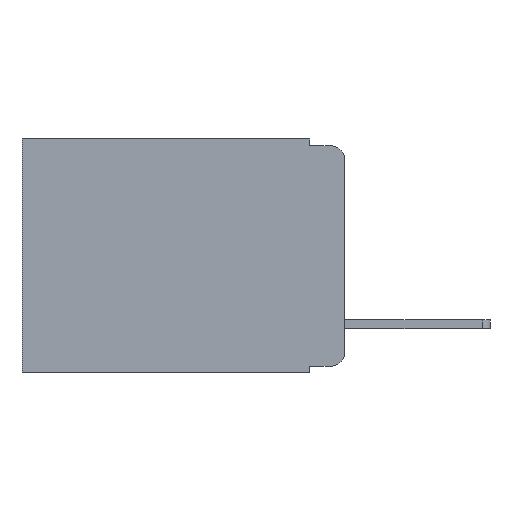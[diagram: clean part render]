
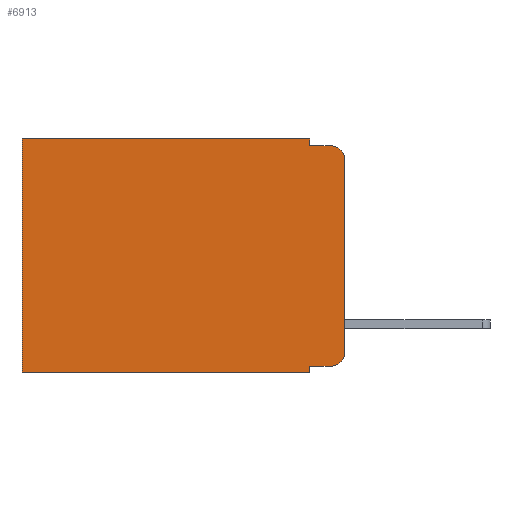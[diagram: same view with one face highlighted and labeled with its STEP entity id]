
A CAD part, left-side view. The second image highlights one B-rep face of the part: STEP entity #6913.
In plain terms, the highlighted planar face has unit normal (-1, 0, 0).
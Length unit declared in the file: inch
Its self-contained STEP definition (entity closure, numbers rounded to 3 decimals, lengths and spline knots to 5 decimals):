
#239 = CARTESIAN_POINT ( 'NONE',  ( 0.298, 0., -0.03 ) ) ;
#267 = VERTEX_POINT ( 'NONE', #1591 ) ;
#398 = CARTESIAN_POINT ( 'NONE',  ( 0.298, 0.473, -0.343 ) ) ;
#424 = DIRECTION ( 'NONE',  ( 0., 1., 0. ) ) ;
#468 = VERTEX_POINT ( 'NONE', #10323 ) ;
#491 = EDGE_CURVE ( 'NONE', #6999, #267, #5347, .T. ) ;
#608 = ORIENTED_EDGE ( 'NONE', *, *, #491, .F. ) ;
#833 = VERTEX_POINT ( 'NONE', #9788 ) ;
#891 = ORIENTED_EDGE ( 'NONE', *, *, #2129, .F. ) ;
#892 = EDGE_CURVE ( 'NONE', #4839, #3375, #2151, .T. ) ;
#1112 = CARTESIAN_POINT ( 'NONE',  ( 0.298, 0., 0. ) ) ;
#1186 = FACE_OUTER_BOUND ( 'NONE', #6972, .T. ) ;
#1490 = ORIENTED_EDGE ( 'NONE', *, *, #1533, .F. ) ;
#1533 = EDGE_CURVE ( 'NONE', #4839, #833, #5191, .T. ) ;
#1591 = CARTESIAN_POINT ( 'NONE',  ( 0.298, 0.051, -0.01 ) ) ;
#1706 = PLANE ( 'NONE',  #8414 ) ;
#1977 = VERTEX_POINT ( 'NONE', #5112 ) ;
#2122 = DIRECTION ( 'NONE',  ( 0., 0., -1. ) ) ;
#2129 = EDGE_CURVE ( 'NONE', #267, #3375, #2554, .T. ) ;
#2151 = CIRCLE ( 'NONE', #7015, 0.02 ) ;
#2209 = CARTESIAN_POINT ( 'NONE',  ( 0.298, 0.051, 0. ) ) ;
#2267 = VECTOR ( 'NONE', #5740, 39.37008 ) ;
#2313 = CARTESIAN_POINT ( 'NONE',  ( 0.298, 0.02, -0.01 ) ) ;
#2428 = EDGE_CURVE ( 'NONE', #1977, #8371, #8918, .T. ) ;
#2472 = AXIS2_PLACEMENT_3D ( 'NONE', #9512, #4552, #10283 ) ;
#2554 = LINE ( 'NONE', #5595, #2267 ) ;
#2742 = CARTESIAN_POINT ( 'NONE',  ( 0.298, 0.051, -0.343 ) ) ;
#2874 = CARTESIAN_POINT ( 'NONE',  ( 0.298, 0., -0.343 ) ) ;
#2921 = LINE ( 'NONE', #2874, #9117 ) ;
#2930 = DIRECTION ( 'NONE',  ( 0., 1., 0. ) ) ;
#3375 = VERTEX_POINT ( 'NONE', #2313 ) ;
#3522 = DIRECTION ( 'NONE',  ( 1., 0., 0. ) ) ;
#3586 = ORIENTED_EDGE ( 'NONE', *, *, #9559, .T. ) ;
#4040 = LINE ( 'NONE', #1112, #6050 ) ;
#4150 = ORIENTED_EDGE ( 'NONE', *, *, #2428, .T. ) ;
#4177 = LINE ( 'NONE', #6265, #5916 ) ;
#4307 = VERTEX_POINT ( 'NONE', #2742 ) ;
#4310 = CARTESIAN_POINT ( 'NONE',  ( 0.298, 0.02, -0.03 ) ) ;
#4516 = DIRECTION ( 'NONE',  ( -1., 0., 0. ) ) ;
#4552 = DIRECTION ( 'NONE',  ( -1., 0., 0. ) ) ;
#4726 = EDGE_CURVE ( 'NONE', #468, #5786, #6727, .T. ) ;
#4756 = VECTOR ( 'NONE', #7923, 39.37008 ) ;
#4793 = EDGE_CURVE ( 'NONE', #468, #4307, #4177, .T. ) ;
#4801 = CIRCLE ( 'NONE', #2472, 0.02 ) ;
#4820 = ORIENTED_EDGE ( 'NONE', *, *, #892, .T. ) ;
#4839 = VERTEX_POINT ( 'NONE', #239 ) ;
#4857 = CARTESIAN_POINT ( 'NONE',  ( 0.298, 0.051, -0.333 ) ) ;
#4916 = VECTOR ( 'NONE', #10443, 39.37008 ) ;
#5079 = VECTOR ( 'NONE', #2122, 39.37008 ) ;
#5112 = CARTESIAN_POINT ( 'NONE',  ( 0.298, 0.473, 0. ) ) ;
#5191 = LINE ( 'NONE', #10582, #4916 ) ;
#5245 = ORIENTED_EDGE ( 'NONE', *, *, #5598, .F. ) ;
#5347 = LINE ( 'NONE', #2209, #5079 ) ;
#5356 = CARTESIAN_POINT ( 'NONE',  ( 0.298, 0.051, 0. ) ) ;
#5595 = CARTESIAN_POINT ( 'NONE',  ( 0.298, 0.051, -0.01 ) ) ;
#5598 = EDGE_CURVE ( 'NONE', #4307, #8371, #2921, .T. ) ;
#5740 = DIRECTION ( 'NONE',  ( 0., -1., 0. ) ) ;
#5786 = VERTEX_POINT ( 'NONE', #8382 ) ;
#5916 = VECTOR ( 'NONE', #6280, 39.37008 ) ;
#6046 = CARTESIAN_POINT ( 'NONE',  ( 0.298, 0., 0. ) ) ;
#6050 = VECTOR ( 'NONE', #2930, 39.37008 ) ;
#6265 = CARTESIAN_POINT ( 'NONE',  ( 0.298, 0.051, 0. ) ) ;
#6280 = DIRECTION ( 'NONE',  ( 0., 0., -1. ) ) ;
#6727 = LINE ( 'NONE', #4857, #8616 ) ;
#6784 = CARTESIAN_POINT ( 'NONE',  ( 0.298, 0.473, 0. ) ) ;
#6913 = ADVANCED_FACE ( 'NONE', ( #1186 ), #1706, .F. ) ;
#6972 = EDGE_LOOP ( 'NONE', ( #1490, #4820, #891, #608, #3586, #4150, #5245, #9341, #9851, #8982 ) ) ;
#6999 = VERTEX_POINT ( 'NONE', #5356 ) ;
#7013 = EDGE_CURVE ( 'NONE', #5786, #833, #4801, .T. ) ;
#7015 = AXIS2_PLACEMENT_3D ( 'NONE', #4310, #4516, #10715 ) ;
#7923 = DIRECTION ( 'NONE',  ( 0., 0., -1. ) ) ;
#8371 = VERTEX_POINT ( 'NONE', #398 ) ;
#8382 = CARTESIAN_POINT ( 'NONE',  ( 0.298, 0.02, -0.333 ) ) ;
#8414 = AXIS2_PLACEMENT_3D ( 'NONE', #6046, #3522, #9370 ) ;
#8616 = VECTOR ( 'NONE', #10179, 39.37008 ) ;
#8918 = LINE ( 'NONE', #6784, #4756 ) ;
#8982 = ORIENTED_EDGE ( 'NONE', *, *, #7013, .T. ) ;
#9117 = VECTOR ( 'NONE', #424, 39.37008 ) ;
#9341 = ORIENTED_EDGE ( 'NONE', *, *, #4793, .F. ) ;
#9370 = DIRECTION ( 'NONE',  ( 0., 0., -1. ) ) ;
#9512 = CARTESIAN_POINT ( 'NONE',  ( 0.298, 0.02, -0.313 ) ) ;
#9559 = EDGE_CURVE ( 'NONE', #6999, #1977, #4040, .T. ) ;
#9788 = CARTESIAN_POINT ( 'NONE',  ( 0.298, 0., -0.313 ) ) ;
#9851 = ORIENTED_EDGE ( 'NONE', *, *, #4726, .T. ) ;
#10179 = DIRECTION ( 'NONE',  ( 0., -1., 0. ) ) ;
#10283 = DIRECTION ( 'NONE',  ( 0., 0., -1. ) ) ;
#10323 = CARTESIAN_POINT ( 'NONE',  ( 0.298, 0.051, -0.333 ) ) ;
#10443 = DIRECTION ( 'NONE',  ( 0., 0., -1. ) ) ;
#10582 = CARTESIAN_POINT ( 'NONE',  ( 0.298, 0., 0. ) ) ;
#10715 = DIRECTION ( 'NONE',  ( 0., 0., -1. ) ) ;
